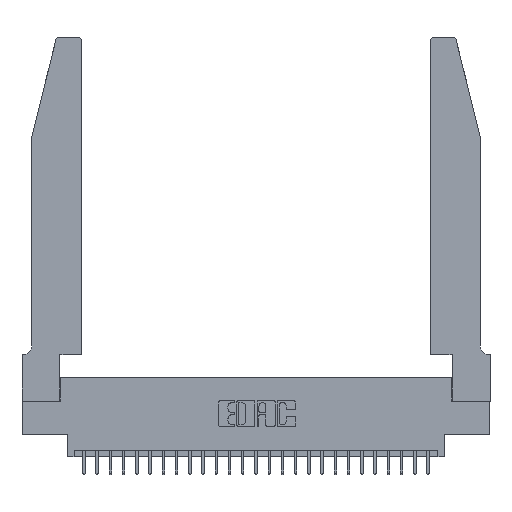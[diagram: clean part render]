
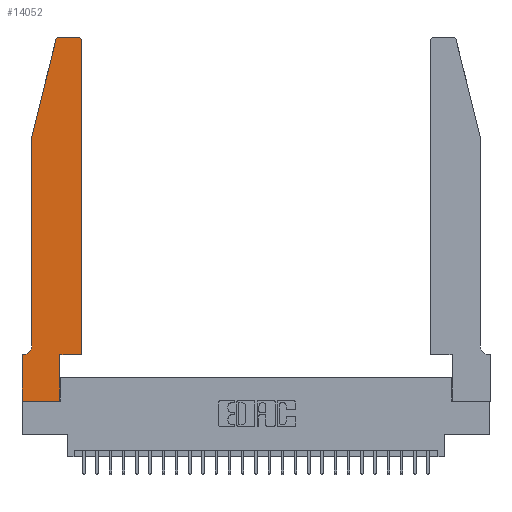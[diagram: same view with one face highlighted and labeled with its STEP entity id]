
A CAD part, top view. The second image highlights one B-rep face of the part: STEP entity #14052.
In plain terms, the highlighted planar face has unit normal (0, 0, 1).
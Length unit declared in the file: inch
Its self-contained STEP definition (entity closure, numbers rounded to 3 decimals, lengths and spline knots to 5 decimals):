
#10 = FACE_OUTER_BOUND ( 'NONE', #26218, .T. ) ;
#282 = DIRECTION ( 'NONE',  ( 0., 0., 1. ) ) ;
#599 = LINE ( 'NONE', #13746, #5359 ) ;
#1100 = VECTOR ( 'NONE', #13932, 39.37008 ) ;
#1220 = CARTESIAN_POINT ( 'NONE',  ( 0., 0., 0.37 ) ) ;
#1610 = ORIENTED_EDGE ( 'NONE', *, *, #15870, .T. ) ;
#1636 = CARTESIAN_POINT ( 'NONE',  ( 0.4505, 0.35, 0.37 ) ) ;
#2289 = VERTEX_POINT ( 'NONE', #5673 ) ;
#2634 = DIRECTION ( 'NONE',  ( -1., 0., 0. ) ) ;
#2655 = VERTEX_POINT ( 'NONE', #13652 ) ;
#2714 = EDGE_CURVE ( 'NONE', #8436, #2289, #18475, .T. ) ;
#2788 = EDGE_CURVE ( 'NONE', #2655, #24909, #5639, .T. ) ;
#3214 = EDGE_CURVE ( 'NONE', #13244, #7146, #5133, .T. ) ;
#3398 = VECTOR ( 'NONE', #10073, 39.37008 ) ;
#3707 = EDGE_CURVE ( 'NONE', #12184, #5269, #5103, .T. ) ;
#3895 = AXIS2_PLACEMENT_3D ( 'NONE', #22412, #5444, #17992 ) ;
#4998 = ORIENTED_EDGE ( 'NONE', *, *, #3214, .T. ) ;
#5041 = VERTEX_POINT ( 'NONE', #18361 ) ;
#5103 = LINE ( 'NONE', #22491, #22542 ) ;
#5133 = LINE ( 'NONE', #22110, #24338 ) ;
#5163 = ORIENTED_EDGE ( 'NONE', *, *, #12552, .T. ) ;
#5269 = VERTEX_POINT ( 'NONE', #25900 ) ;
#5359 = VECTOR ( 'NONE', #7322, 39.37008 ) ;
#5444 = DIRECTION ( 'NONE',  ( 0., 0., 1. ) ) ;
#5631 = VERTEX_POINT ( 'NONE', #6220 ) ;
#5639 = LINE ( 'NONE', #1636, #3398 ) ;
#5673 = CARTESIAN_POINT ( 'NONE',  ( 0., 0., 0.37 ) ) ;
#6220 = CARTESIAN_POINT ( 'NONE',  ( 0.25487, 2.72718, 0.37 ) ) ;
#6904 = CARTESIAN_POINT ( 'NONE',  ( 0.0055, 0.42, 0.37 ) ) ;
#7146 = VERTEX_POINT ( 'NONE', #20844 ) ;
#7179 = LINE ( 'NONE', #13741, #9138 ) ;
#7322 = DIRECTION ( 'NONE',  ( -0.239, -0.971, 0. ) ) ;
#7442 = DIRECTION ( 'NONE',  ( 1., 0., 0. ) ) ;
#8436 = VERTEX_POINT ( 'NONE', #22836 ) ;
#8896 = EDGE_CURVE ( 'NONE', #10867, #5041, #22798, .T. ) ;
#9120 = AXIS2_PLACEMENT_3D ( 'NONE', #20321, #16043, #24727 ) ;
#9138 = VECTOR ( 'NONE', #22416, 39.37008 ) ;
#9564 = CIRCLE ( 'NONE', #9120, 0.03 ) ;
#9588 = CIRCLE ( 'NONE', #25508, 0.07 ) ;
#9666 = DIRECTION ( 'NONE',  ( -1., 0., 0. ) ) ;
#10014 = VERTEX_POINT ( 'NONE', #24797 ) ;
#10073 = DIRECTION ( 'NONE',  ( 0., 1., 0. ) ) ;
#10867 = VERTEX_POINT ( 'NONE', #19895 ) ;
#11198 = EDGE_CURVE ( 'NONE', #5041, #2655, #26523, .T. ) ;
#11296 = CARTESIAN_POINT ( 'NONE',  ( 0.4505, 0.35, 0.37 ) ) ;
#11966 = CARTESIAN_POINT ( 'NONE',  ( 0.2865, 0.35, 0.37 ) ) ;
#12184 = VERTEX_POINT ( 'NONE', #22443 ) ;
#12552 = EDGE_CURVE ( 'NONE', #24909, #13244, #28025, .T. ) ;
#13059 = ORIENTED_EDGE ( 'NONE', *, *, #11198, .T. ) ;
#13118 = ORIENTED_EDGE ( 'NONE', *, *, #20129, .T. ) ;
#13244 = VERTEX_POINT ( 'NONE', #23645 ) ;
#13652 = CARTESIAN_POINT ( 'NONE',  ( 0.4505, 0.35, 0.37 ) ) ;
#13741 = CARTESIAN_POINT ( 'NONE',  ( 0., 0., 0.37 ) ) ;
#13746 = CARTESIAN_POINT ( 'NONE',  ( 0.0755, 2., 0.37 ) ) ;
#13811 = DIRECTION ( 'NONE',  ( 0., -1., 0. ) ) ;
#13932 = DIRECTION ( 'NONE',  ( 0., -1., 0. ) ) ;
#14052 = ADVANCED_FACE ( 'NONE', ( #10 ), #21557, .T. ) ;
#15493 = ORIENTED_EDGE ( 'NONE', *, *, #3707, .T. ) ;
#15560 = DIRECTION ( 'NONE',  ( 1., 0., 0. ) ) ;
#15870 = EDGE_CURVE ( 'NONE', #10014, #8436, #18079, .T. ) ;
#16010 = ORIENTED_EDGE ( 'NONE', *, *, #2788, .T. ) ;
#16043 = DIRECTION ( 'NONE',  ( 0., 0., 1. ) ) ;
#16115 = DIRECTION ( 'NONE',  ( -1., 0., 0. ) ) ;
#16811 = EDGE_CURVE ( 'NONE', #5631, #12184, #599, .T. ) ;
#17992 = DIRECTION ( 'NONE',  ( 1., 0., 0. ) ) ;
#18079 = LINE ( 'NONE', #24911, #27139 ) ;
#18361 = CARTESIAN_POINT ( 'NONE',  ( 0.2865, 0.35, 0.37 ) ) ;
#18442 = ORIENTED_EDGE ( 'NONE', *, *, #27821, .T. ) ;
#18461 = ORIENTED_EDGE ( 'NONE', *, *, #8896, .T. ) ;
#18475 = LINE ( 'NONE', #1220, #1100 ) ;
#19860 = AXIS2_PLACEMENT_3D ( 'NONE', #26089, #282, #15560 ) ;
#19895 = CARTESIAN_POINT ( 'NONE',  ( 0.2865, 0., 0.37 ) ) ;
#20129 = EDGE_CURVE ( 'NONE', #7146, #5631, #9564, .T. ) ;
#20321 = CARTESIAN_POINT ( 'NONE',  ( 0.284, 2.72, 0.37 ) ) ;
#20646 = EDGE_CURVE ( 'NONE', #2289, #10867, #7179, .T. ) ;
#20844 = CARTESIAN_POINT ( 'NONE',  ( 0.284, 2.75, 0.37 ) ) ;
#21557 = PLANE ( 'NONE',  #19860 ) ;
#21587 = VECTOR ( 'NONE', #7442, 39.37008 ) ;
#22110 = CARTESIAN_POINT ( 'NONE',  ( 0.2605, 2.75, 0.37 ) ) ;
#22161 = DIRECTION ( 'NONE',  ( 0., 0., -1. ) ) ;
#22326 = ORIENTED_EDGE ( 'NONE', *, *, #16811, .T. ) ;
#22412 = CARTESIAN_POINT ( 'NONE',  ( 0.4205, 2.72, 0.37 ) ) ;
#22416 = DIRECTION ( 'NONE',  ( 1., 0., 0. ) ) ;
#22443 = CARTESIAN_POINT ( 'NONE',  ( 0.0755, 2., 0.37 ) ) ;
#22491 = CARTESIAN_POINT ( 'NONE',  ( 0.0755, 2., 0.37 ) ) ;
#22542 = VECTOR ( 'NONE', #13811, 39.37008 ) ;
#22798 = LINE ( 'NONE', #11966, #23446 ) ;
#22836 = CARTESIAN_POINT ( 'NONE',  ( 0., 0.35, 0.37 ) ) ;
#23215 = DIRECTION ( 'NONE',  ( 0., 1., 0. ) ) ;
#23446 = VECTOR ( 'NONE', #23215, 39.37008 ) ;
#23645 = CARTESIAN_POINT ( 'NONE',  ( 0.4205, 2.75, 0.37 ) ) ;
#24338 = VECTOR ( 'NONE', #16115, 39.37008 ) ;
#24727 = DIRECTION ( 'NONE',  ( 1., 0., 0. ) ) ;
#24764 = CARTESIAN_POINT ( 'NONE',  ( 0.4505, 2.72, 0.37 ) ) ;
#24797 = CARTESIAN_POINT ( 'NONE',  ( 0.0055, 0.35, 0.37 ) ) ;
#24909 = VERTEX_POINT ( 'NONE', #24764 ) ;
#24911 = CARTESIAN_POINT ( 'NONE',  ( 0.0755, 0.35, 0.37 ) ) ;
#25100 = ORIENTED_EDGE ( 'NONE', *, *, #20646, .T. ) ;
#25508 = AXIS2_PLACEMENT_3D ( 'NONE', #6904, #22161, #2634 ) ;
#25900 = CARTESIAN_POINT ( 'NONE',  ( 0.0755, 0.42, 0.37 ) ) ;
#26089 = CARTESIAN_POINT ( 'NONE',  ( 0., 0.35, 0.37 ) ) ;
#26218 = EDGE_LOOP ( 'NONE', ( #4998, #13118, #22326, #15493, #18442, #1610, #27246, #25100, #18461, #13059, #16010, #5163 ) ) ;
#26523 = LINE ( 'NONE', #11296, #21587 ) ;
#27139 = VECTOR ( 'NONE', #9666, 39.37008 ) ;
#27246 = ORIENTED_EDGE ( 'NONE', *, *, #2714, .T. ) ;
#27821 = EDGE_CURVE ( 'NONE', #5269, #10014, #9588, .T. ) ;
#28025 = CIRCLE ( 'NONE', #3895, 0.03 ) ;
